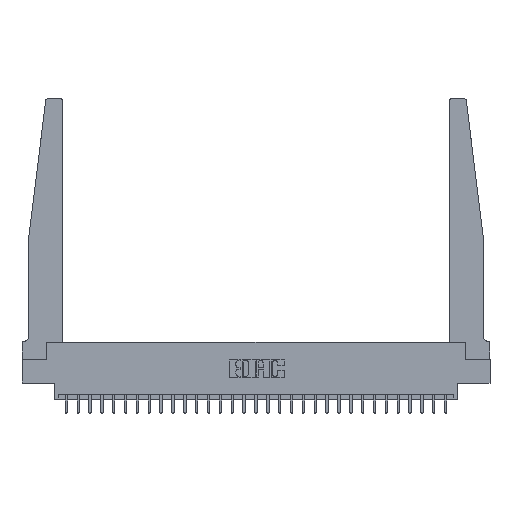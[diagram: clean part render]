
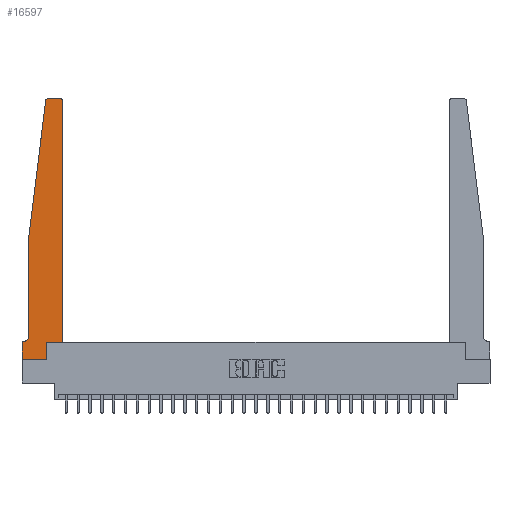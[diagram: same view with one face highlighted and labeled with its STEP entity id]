
A CAD part, top view. The second image highlights one B-rep face of the part: STEP entity #16597.
In plain terms, the highlighted planar face has unit normal (0, 0, 1).
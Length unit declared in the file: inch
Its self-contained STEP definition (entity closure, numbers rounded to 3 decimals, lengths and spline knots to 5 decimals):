
#198 = CARTESIAN_POINT ( 'NONE',  ( 0.395, 2.72, 0.37 ) ) ;
#318 = CARTESIAN_POINT ( 'NONE',  ( 0.065, 1.25, 0.37 ) ) ;
#366 = VECTOR ( 'NONE', #24312, 39.37008 ) ;
#479 = VERTEX_POINT ( 'NONE', #16585 ) ;
#1138 = DIRECTION ( 'NONE',  ( 0., 0., 1. ) ) ;
#1289 = VERTEX_POINT ( 'NONE', #6098 ) ;
#1459 = CARTESIAN_POINT ( 'NONE',  ( 0.24675, 2.72367, 0.37 ) ) ;
#1614 = ORIENTED_EDGE ( 'NONE', *, *, #18168, .T. ) ;
#1646 = VECTOR ( 'NONE', #17205, 39.37008 ) ;
#1846 = VERTEX_POINT ( 'NONE', #8860 ) ;
#1991 = CARTESIAN_POINT ( 'NONE',  ( 0.25, 2.75, 0.37 ) ) ;
#2439 = DIRECTION ( 'NONE',  ( -1., 0., 0. ) ) ;
#3093 = ORIENTED_EDGE ( 'NONE', *, *, #9566, .T. ) ;
#3378 = CIRCLE ( 'NONE', #19294, 0.05 ) ;
#3427 = VERTEX_POINT ( 'NONE', #24950 ) ;
#4151 = DIRECTION ( 'NONE',  ( 1., 0., 0. ) ) ;
#4251 = CARTESIAN_POINT ( 'NONE',  ( 0., 0.1875, 0.37 ) ) ;
#5160 = VERTEX_POINT ( 'NONE', #11518 ) ;
#5776 = CARTESIAN_POINT ( 'NONE',  ( 0.015, 0.1875, 0.37 ) ) ;
#5794 = PLANE ( 'NONE',  #27011 ) ;
#6098 = CARTESIAN_POINT ( 'NONE',  ( 0., 0., 0.37 ) ) ;
#6234 = VECTOR ( 'NONE', #17341, 39.37008 ) ;
#6485 = VECTOR ( 'NONE', #22052, 39.37008 ) ;
#6791 = CARTESIAN_POINT ( 'NONE',  ( 0.425, 0.18, 0.37 ) ) ;
#6807 = EDGE_CURVE ( 'NONE', #15755, #5160, #13672, .T. ) ;
#7065 = DIRECTION ( 'NONE',  ( 1., 0., 0. ) ) ;
#8176 = ORIENTED_EDGE ( 'NONE', *, *, #19555, .T. ) ;
#8407 = VECTOR ( 'NONE', #26170, 39.37008 ) ;
#8431 = VECTOR ( 'NONE', #18386, 39.37008 ) ;
#8473 = VERTEX_POINT ( 'NONE', #4251 ) ;
#8622 = EDGE_CURVE ( 'NONE', #5160, #10531, #11479, .T. ) ;
#8860 = CARTESIAN_POINT ( 'NONE',  ( 0.27653, 2.75, 0.37 ) ) ;
#9459 = CARTESIAN_POINT ( 'NONE',  ( 0.425, 2.72, 0.37 ) ) ;
#9566 = EDGE_CURVE ( 'NONE', #14572, #8473, #27086, .T. ) ;
#9725 = VECTOR ( 'NONE', #18726, 39.37008 ) ;
#10168 = LINE ( 'NONE', #14185, #9725 ) ;
#10531 = VERTEX_POINT ( 'NONE', #9459 ) ;
#11133 = EDGE_CURVE ( 'NONE', #479, #1846, #17052, .T. ) ;
#11144 = EDGE_CURVE ( 'NONE', #17938, #27492, #23884, .T. ) ;
#11352 = LINE ( 'NONE', #24313, #23731 ) ;
#11422 = ORIENTED_EDGE ( 'NONE', *, *, #26790, .T. ) ;
#11479 = LINE ( 'NONE', #6791, #366 ) ;
#11518 = CARTESIAN_POINT ( 'NONE',  ( 0.425, 0.18, 0.37 ) ) ;
#11817 = EDGE_LOOP ( 'NONE', ( #15714, #1614, #21429, #11422, #8176, #3093, #22708, #19609, #20701, #12178, #16244, #19288 ) ) ;
#12178 = ORIENTED_EDGE ( 'NONE', *, *, #6807, .T. ) ;
#12783 = LINE ( 'NONE', #26029, #6234 ) ;
#13236 = CARTESIAN_POINT ( 'NONE',  ( 0.015, 0.2375, 0.37 ) ) ;
#13672 = LINE ( 'NONE', #19932, #6485 ) ;
#14185 = CARTESIAN_POINT ( 'NONE',  ( 0., 0., 0.37 ) ) ;
#14299 = EDGE_CURVE ( 'NONE', #1289, #25312, #11352, .T. ) ;
#14358 = CARTESIAN_POINT ( 'NONE',  ( 0., 0.1875, 0.37 ) ) ;
#14572 = VERTEX_POINT ( 'NONE', #5776 ) ;
#15249 = CIRCLE ( 'NONE', #17510, 0.03 ) ;
#15416 = AXIS2_PLACEMENT_3D ( 'NONE', #198, #20842, #4151 ) ;
#15714 = ORIENTED_EDGE ( 'NONE', *, *, #11133, .T. ) ;
#15755 = VERTEX_POINT ( 'NONE', #15901 ) ;
#15901 = CARTESIAN_POINT ( 'NONE',  ( 0.2605, 0.18, 0.37 ) ) ;
#16244 = ORIENTED_EDGE ( 'NONE', *, *, #8622, .T. ) ;
#16585 = CARTESIAN_POINT ( 'NONE',  ( 0.395, 2.75, 0.37 ) ) ;
#16597 = ADVANCED_FACE ( 'NONE', ( #25314 ), #5794, .T. ) ;
#17052 = LINE ( 'NONE', #1991, #8407 ) ;
#17097 = EDGE_CURVE ( 'NONE', #8473, #1289, #10168, .T. ) ;
#17205 = DIRECTION ( 'NONE',  ( -0.122, -0.992, 0. ) ) ;
#17341 = DIRECTION ( 'NONE',  ( 0., 1., 0. ) ) ;
#17510 = AXIS2_PLACEMENT_3D ( 'NONE', #21358, #20030, #26739 ) ;
#17878 = CARTESIAN_POINT ( 'NONE',  ( 0.065, 1.25, 0.37 ) ) ;
#17938 = VERTEX_POINT ( 'NONE', #1459 ) ;
#18168 = EDGE_CURVE ( 'NONE', #1846, #17938, #15249, .T. ) ;
#18386 = DIRECTION ( 'NONE',  ( -1., 0., 0. ) ) ;
#18726 = DIRECTION ( 'NONE',  ( 0., -1., 0. ) ) ;
#18761 = DIRECTION ( 'NONE',  ( 1., 0., 0. ) ) ;
#19288 = ORIENTED_EDGE ( 'NONE', *, *, #24412, .T. ) ;
#19294 = AXIS2_PLACEMENT_3D ( 'NONE', #13236, #28066, #2439 ) ;
#19555 = EDGE_CURVE ( 'NONE', #3427, #14572, #3378, .T. ) ;
#19609 = ORIENTED_EDGE ( 'NONE', *, *, #14299, .T. ) ;
#19932 = CARTESIAN_POINT ( 'NONE',  ( 0.425, 0.18, 0.37 ) ) ;
#20030 = DIRECTION ( 'NONE',  ( 0., 0., 1. ) ) ;
#20701 = ORIENTED_EDGE ( 'NONE', *, *, #22449, .T. ) ;
#20842 = DIRECTION ( 'NONE',  ( 0., 0., 1. ) ) ;
#21358 = CARTESIAN_POINT ( 'NONE',  ( 0.27653, 2.72, 0.37 ) ) ;
#21429 = ORIENTED_EDGE ( 'NONE', *, *, #11144, .T. ) ;
#21878 = CARTESIAN_POINT ( 'NONE',  ( 0.065, 1.25, 0.37 ) ) ;
#22001 = LINE ( 'NONE', #17878, #24073 ) ;
#22052 = DIRECTION ( 'NONE',  ( 1., 0., 0. ) ) ;
#22449 = EDGE_CURVE ( 'NONE', #25312, #15755, #12783, .T. ) ;
#22708 = ORIENTED_EDGE ( 'NONE', *, *, #17097, .T. ) ;
#22792 = CARTESIAN_POINT ( 'NONE',  ( 0.065, 0.1875, 0.37 ) ) ;
#23731 = VECTOR ( 'NONE', #7065, 39.37008 ) ;
#23884 = LINE ( 'NONE', #21878, #1646 ) ;
#24073 = VECTOR ( 'NONE', #26575, 39.37008 ) ;
#24312 = DIRECTION ( 'NONE',  ( 0., 1., 0. ) ) ;
#24313 = CARTESIAN_POINT ( 'NONE',  ( 0., 0., 0.37 ) ) ;
#24412 = EDGE_CURVE ( 'NONE', #10531, #479, #24514, .T. ) ;
#24514 = CIRCLE ( 'NONE', #15416, 0.03 ) ;
#24950 = CARTESIAN_POINT ( 'NONE',  ( 0.065, 0.2375, 0.37 ) ) ;
#25312 = VERTEX_POINT ( 'NONE', #27313 ) ;
#25314 = FACE_OUTER_BOUND ( 'NONE', #11817, .T. ) ;
#26029 = CARTESIAN_POINT ( 'NONE',  ( 0.2605, 0.18, 0.37 ) ) ;
#26170 = DIRECTION ( 'NONE',  ( -1., 0., 0. ) ) ;
#26575 = DIRECTION ( 'NONE',  ( 0., -1., 0. ) ) ;
#26739 = DIRECTION ( 'NONE',  ( 1., 0., 0. ) ) ;
#26790 = EDGE_CURVE ( 'NONE', #27492, #3427, #22001, .T. ) ;
#27011 = AXIS2_PLACEMENT_3D ( 'NONE', #14358, #1138, #18761 ) ;
#27086 = LINE ( 'NONE', #22792, #8431 ) ;
#27313 = CARTESIAN_POINT ( 'NONE',  ( 0.2605, 0., 0.37 ) ) ;
#27492 = VERTEX_POINT ( 'NONE', #318 ) ;
#28066 = DIRECTION ( 'NONE',  ( 0., 0., -1. ) ) ;
